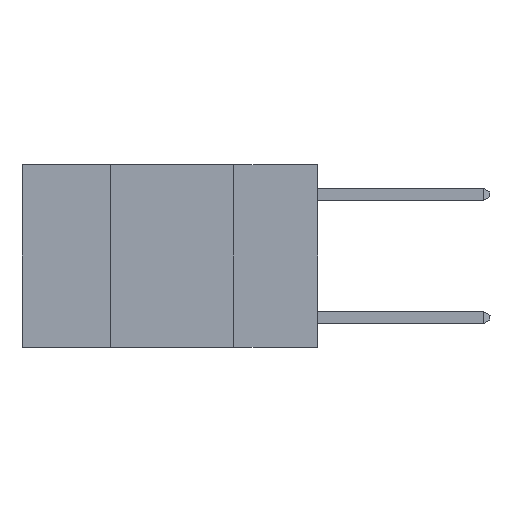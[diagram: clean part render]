
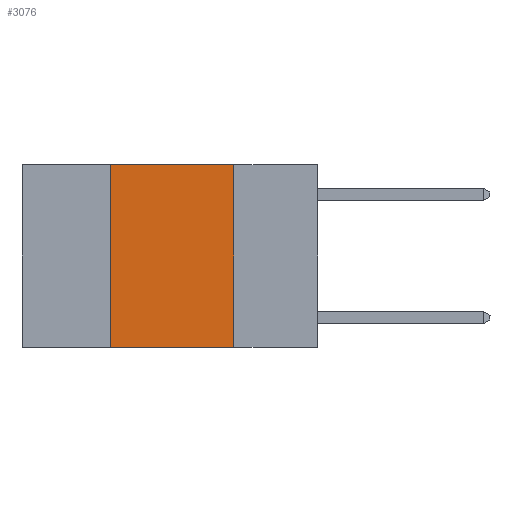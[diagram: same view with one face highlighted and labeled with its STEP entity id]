
A CAD part, left-side view. The second image highlights one B-rep face of the part: STEP entity #3076.
In plain terms, the highlighted planar face has unit normal (-1, 0, 0).
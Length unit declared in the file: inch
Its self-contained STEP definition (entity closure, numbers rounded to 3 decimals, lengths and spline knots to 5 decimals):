
#778 = ORIENTED_EDGE ( 'NONE', *, *, #8309, .F. ) ;
#938 = EDGE_CURVE ( 'NONE', #2458, #4065, #6104, .T. ) ;
#1025 = LINE ( 'NONE', #9160, #9158 ) ;
#1291 = DIRECTION ( 'NONE',  ( 0., -1., 0. ) ) ;
#1499 = VECTOR ( 'NONE', #7792, 39.37008 ) ;
#1684 = VERTEX_POINT ( 'NONE', #8580 ) ;
#1860 = FACE_OUTER_BOUND ( 'NONE', #1953, .T. ) ;
#1953 = EDGE_LOOP ( 'NONE', ( #5061, #7091, #778, #7309 ) ) ;
#2124 = DIRECTION ( 'NONE',  ( 0., 0., 1. ) ) ;
#2458 = VERTEX_POINT ( 'NONE', #10070 ) ;
#2571 = CARTESIAN_POINT ( 'NONE',  ( 0., 0.6, 0. ) ) ;
#3076 = ADVANCED_FACE ( 'NONE', ( #1860 ), #8714, .F. ) ;
#3098 = VERTEX_POINT ( 'NONE', #8023 ) ;
#3662 = LINE ( 'NONE', #6227, #3927 ) ;
#3927 = VECTOR ( 'NONE', #1291, 39.37008 ) ;
#4065 = VERTEX_POINT ( 'NONE', #8818 ) ;
#4380 = VECTOR ( 'NONE', #2124, 39.37008 ) ;
#5061 = ORIENTED_EDGE ( 'NONE', *, *, #8485, .F. ) ;
#5539 = AXIS2_PLACEMENT_3D ( 'NONE', #2571, #9420, #9452 ) ;
#5752 = EDGE_CURVE ( 'NONE', #3098, #1684, #3662, .T. ) ;
#6104 = LINE ( 'NONE', #9006, #1499 ) ;
#6227 = CARTESIAN_POINT ( 'NONE',  ( 0., 0.6, -0.37 ) ) ;
#6439 = LINE ( 'NONE', #9767, #4380 ) ;
#7091 = ORIENTED_EDGE ( 'NONE', *, *, #938, .F. ) ;
#7309 = ORIENTED_EDGE ( 'NONE', *, *, #5752, .T. ) ;
#7792 = DIRECTION ( 'NONE',  ( 0., -1., 0. ) ) ;
#8023 = CARTESIAN_POINT ( 'NONE',  ( 0., 0.42, -0.37 ) ) ;
#8309 = EDGE_CURVE ( 'NONE', #3098, #2458, #6439, .T. ) ;
#8485 = EDGE_CURVE ( 'NONE', #4065, #1684, #1025, .T. ) ;
#8580 = CARTESIAN_POINT ( 'NONE',  ( 0., 0.17, -0.37 ) ) ;
#8714 = PLANE ( 'NONE',  #5539 ) ;
#8818 = CARTESIAN_POINT ( 'NONE',  ( 0., 0.17, 0. ) ) ;
#9006 = CARTESIAN_POINT ( 'NONE',  ( 0., 0.6, 0. ) ) ;
#9158 = VECTOR ( 'NONE', #9900, 39.37008 ) ;
#9160 = CARTESIAN_POINT ( 'NONE',  ( 0., 0.17, 0. ) ) ;
#9420 = DIRECTION ( 'NONE',  ( 1., 0., 0. ) ) ;
#9452 = DIRECTION ( 'NONE',  ( 0., 0., -1. ) ) ;
#9767 = CARTESIAN_POINT ( 'NONE',  ( 0., 0.42, 0. ) ) ;
#9900 = DIRECTION ( 'NONE',  ( 0., 0., -1. ) ) ;
#10070 = CARTESIAN_POINT ( 'NONE',  ( 0., 0.42, 0. ) ) ;
